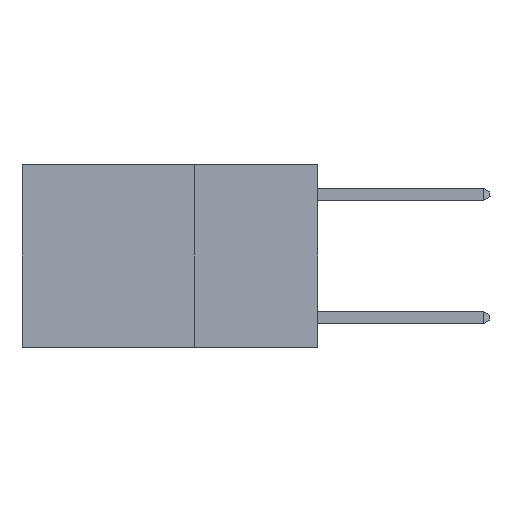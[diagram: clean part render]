
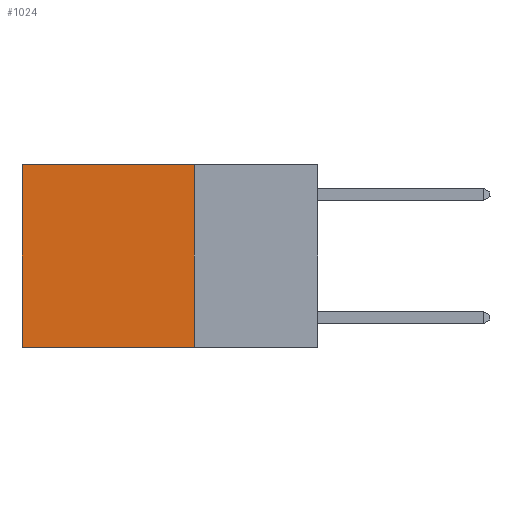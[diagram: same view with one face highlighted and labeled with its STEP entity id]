
A CAD part, left-side view. The second image highlights one B-rep face of the part: STEP entity #1024.
In plain terms, the highlighted planar face has unit normal (-1, 0, 0).
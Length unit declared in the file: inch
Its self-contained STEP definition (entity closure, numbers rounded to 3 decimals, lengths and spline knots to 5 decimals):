
#108 = CARTESIAN_POINT ( 'NONE',  ( 0.2625, 0.25, -0.37 ) ) ;
#451 = ORIENTED_EDGE ( 'NONE', *, *, #4782, .F. ) ;
#617 = DIRECTION ( 'NONE',  ( 0., 1., 0. ) ) ;
#1024 = ADVANCED_FACE ( 'NONE', ( #4539 ), #2915, .F. ) ;
#1352 = CARTESIAN_POINT ( 'NONE',  ( 0.2625, 0.25, -0.37 ) ) ;
#1645 = CARTESIAN_POINT ( 'NONE',  ( 0.2625, 0.25, 0. ) ) ;
#1663 = EDGE_LOOP ( 'NONE', ( #5704, #451, #8946, #7241 ) ) ;
#2690 = VECTOR ( 'NONE', #5937, 39.37008 ) ;
#2915 = PLANE ( 'NONE',  #8609 ) ;
#3091 = DIRECTION ( 'NONE',  ( 0., 0., -1. ) ) ;
#3106 = CARTESIAN_POINT ( 'NONE',  ( 0.2625, 0.25, 0. ) ) ;
#3627 = CARTESIAN_POINT ( 'NONE',  ( 0.2625, 0.25, 0. ) ) ;
#3709 = CARTESIAN_POINT ( 'NONE',  ( 0.2625, 0.6, 0. ) ) ;
#3810 = VECTOR ( 'NONE', #4653, 39.37008 ) ;
#4360 = CARTESIAN_POINT ( 'NONE',  ( 0.2625, 0.25, 0. ) ) ;
#4539 = FACE_OUTER_BOUND ( 'NONE', #1663, .T. ) ;
#4653 = DIRECTION ( 'NONE',  ( 0., 1., 0. ) ) ;
#4669 = LINE ( 'NONE', #8359, #8998 ) ;
#4683 = EDGE_CURVE ( 'NONE', #7922, #9586, #8736, .T. ) ;
#4782 = EDGE_CURVE ( 'NONE', #9586, #5361, #9527, .T. ) ;
#5238 = CARTESIAN_POINT ( 'NONE',  ( 0.2625, 0.6, -0.37 ) ) ;
#5280 = DIRECTION ( 'NONE',  ( 1., 0., 0. ) ) ;
#5361 = VERTEX_POINT ( 'NONE', #5238 ) ;
#5395 = LINE ( 'NONE', #1645, #3810 ) ;
#5704 = ORIENTED_EDGE ( 'NONE', *, *, #7663, .T. ) ;
#5926 = DIRECTION ( 'NONE',  ( 0., 0., -1. ) ) ;
#5937 = DIRECTION ( 'NONE',  ( 0., 0., -1. ) ) ;
#6337 = EDGE_CURVE ( 'NONE', #7922, #7150, #5395, .T. ) ;
#7150 = VERTEX_POINT ( 'NONE', #3709 ) ;
#7241 = ORIENTED_EDGE ( 'NONE', *, *, #6337, .T. ) ;
#7414 = VECTOR ( 'NONE', #617, 39.37008 ) ;
#7663 = EDGE_CURVE ( 'NONE', #7150, #5361, #4669, .T. ) ;
#7922 = VERTEX_POINT ( 'NONE', #3627 ) ;
#8359 = CARTESIAN_POINT ( 'NONE',  ( 0.2625, 0.6, 0. ) ) ;
#8609 = AXIS2_PLACEMENT_3D ( 'NONE', #3106, #5280, #5926 ) ;
#8736 = LINE ( 'NONE', #4360, #2690 ) ;
#8946 = ORIENTED_EDGE ( 'NONE', *, *, #4683, .F. ) ;
#8998 = VECTOR ( 'NONE', #3091, 39.37008 ) ;
#9527 = LINE ( 'NONE', #1352, #7414 ) ;
#9586 = VERTEX_POINT ( 'NONE', #108 ) ;
